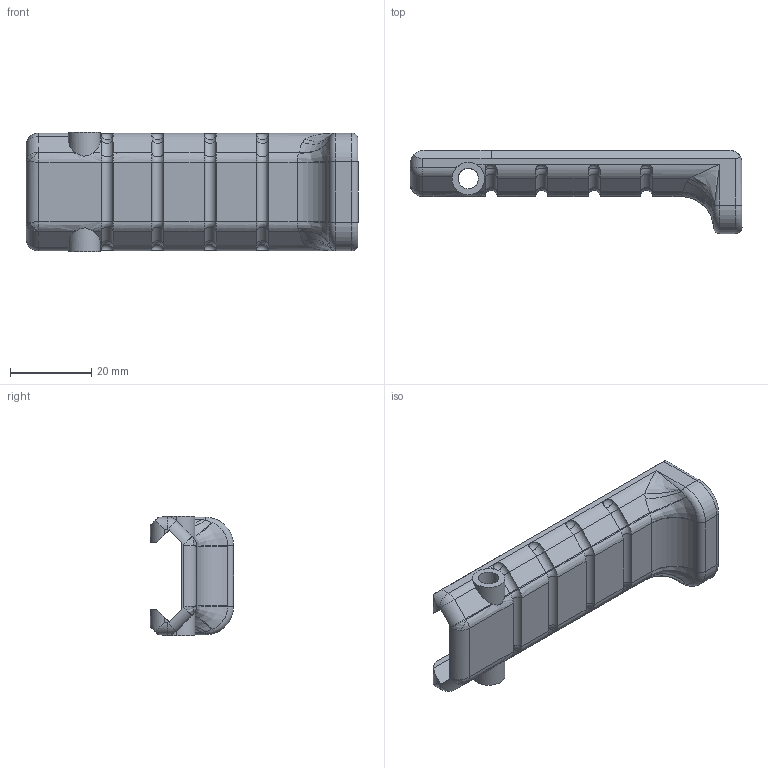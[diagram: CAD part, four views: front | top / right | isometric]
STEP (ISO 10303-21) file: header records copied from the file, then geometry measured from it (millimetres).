
FILE_DESCRIPTION(/* description */ (''),/* implementation_level */ '2;1');
FILE_NAME(/* name */ 'vz61 Handstop.step',/* time_stamp */ '2021-02-09T08:47:33-07:00',/* author */ (''),/* organization */ (''),/* preprocessor_version */ 'ST-DEVELOPER v18.1',/* originating_system */ 'Autodesk Translation Framework v9.7.1.1290',/* authorisation */ '');
FILE_SCHEMA (('AUTOMOTIVE_DESIGN { 1 0 10303 214 3 1 1 }'));
Length unit declared in the file: millimetre
Products named in the file (1): vz61 Handguard
Bounding box: 81.82 x 20.5 x 29.54 mm (x, y, z)
Volume: 13343 mm3; surface area: 8623.3 mm2
Topology: 1 solids, 1 shells, 208 faces, 526 edges, 313 vertices
Faces by surface type: plane 64, bspline 57, cylinder 57, torus 20, sphere 10
Full cylindrical faces by diameter (mm): 5.045 x2
Entity records: 7904 total; most frequent: CARTESIAN_POINT 3310, ORIENTED_EDGE 1042, DIRECTION 808, EDGE_CURVE 521, VERTEX_POINT 313, AXIS2_PLACEMENT_3D 306, EDGE_LOOP 210, FACE_OUTER_BOUND 208
